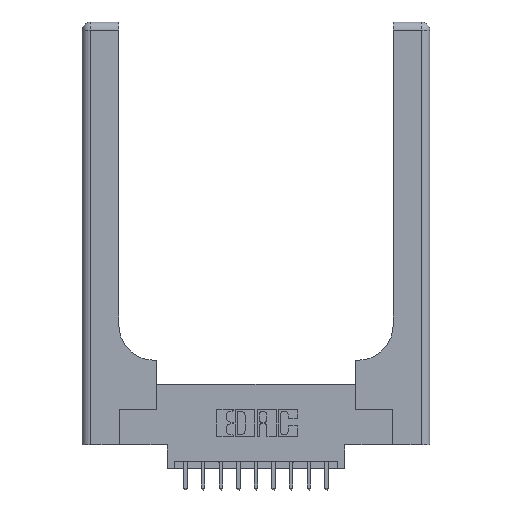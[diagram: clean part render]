
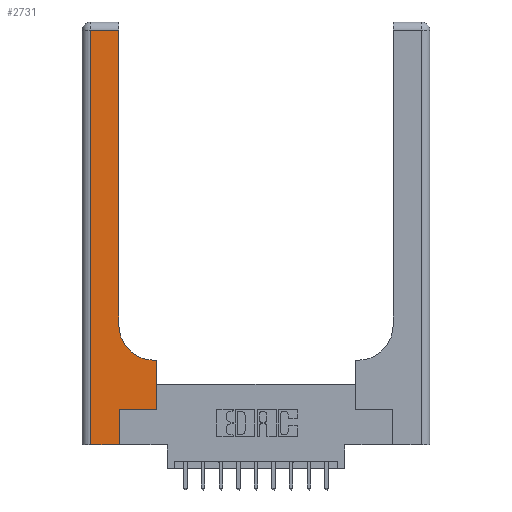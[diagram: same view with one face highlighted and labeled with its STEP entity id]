
A CAD part, top view. The second image highlights one B-rep face of the part: STEP entity #2731.
In plain terms, the highlighted planar face has unit normal (0, 0, 1).
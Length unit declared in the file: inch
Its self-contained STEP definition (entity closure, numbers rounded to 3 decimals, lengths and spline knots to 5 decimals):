
#89 = DIRECTION ( 'NONE',  ( 1., 0., 0. ) ) ;
#247 = CARTESIAN_POINT ( 'NONE',  ( 0.51, 0.85, 0.37 ) ) ;
#337 = VECTOR ( 'NONE', #2389, 39.37008 ) ;
#492 = LINE ( 'NONE', #6686, #12989 ) ;
#712 = EDGE_CURVE ( 'NONE', #7349, #15351, #12527, .T. ) ;
#762 = EDGE_CURVE ( 'NONE', #5859, #15444, #8938, .T. ) ;
#1408 = VECTOR ( 'NONE', #10442, 39.37008 ) ;
#1479 = CARTESIAN_POINT ( 'NONE',  ( 0.265, 0.25, 0.37 ) ) ;
#1550 = LINE ( 'NONE', #6518, #12746 ) ;
#1628 = VECTOR ( 'NONE', #10162, 39.37008 ) ;
#1640 = LINE ( 'NONE', #9027, #1628 ) ;
#1655 = ORIENTED_EDGE ( 'NONE', *, *, #3115, .T. ) ;
#1738 = VERTEX_POINT ( 'NONE', #7771 ) ;
#1803 = LINE ( 'NONE', #6767, #12685 ) ;
#2389 = DIRECTION ( 'NONE',  ( 0., 1., 0. ) ) ;
#2731 = ADVANCED_FACE ( 'NONE', ( #12459 ), #4994, .F. ) ;
#3050 = ORIENTED_EDGE ( 'NONE', *, *, #10567, .T. ) ;
#3115 = EDGE_CURVE ( 'NONE', #15982, #5859, #492, .T. ) ;
#3311 = LINE ( 'NONE', #5437, #1408 ) ;
#3332 = ORIENTED_EDGE ( 'NONE', *, *, #15633, .T. ) ;
#3412 = ORIENTED_EDGE ( 'NONE', *, *, #13233, .T. ) ;
#4410 = VERTEX_POINT ( 'NONE', #16093 ) ;
#4531 = ORIENTED_EDGE ( 'NONE', *, *, #712, .T. ) ;
#4686 = ORIENTED_EDGE ( 'NONE', *, *, #762, .T. ) ;
#4962 = AXIS2_PLACEMENT_3D ( 'NONE', #8559, #8634, #7187 ) ;
#4994 = PLANE ( 'NONE',  #4962 ) ;
#5211 = LINE ( 'NONE', #6184, #6594 ) ;
#5437 = CARTESIAN_POINT ( 'NONE',  ( 0.528, 0.25, 0.37 ) ) ;
#5447 = EDGE_CURVE ( 'NONE', #1738, #7543, #1803, .T. ) ;
#5859 = VERTEX_POINT ( 'NONE', #10223 ) ;
#5895 = CARTESIAN_POINT ( 'NONE',  ( 0.265, 0., 0.37 ) ) ;
#6066 = ORIENTED_EDGE ( 'NONE', *, *, #5447, .T. ) ;
#6184 = CARTESIAN_POINT ( 'NONE',  ( 0., 2.94, 0.37 ) ) ;
#6518 = CARTESIAN_POINT ( 'NONE',  ( 0.26, 3., 0.37 ) ) ;
#6594 = VECTOR ( 'NONE', #10142, 39.37008 ) ;
#6686 = CARTESIAN_POINT ( 'NONE',  ( 0.26, 0.6, 0.37 ) ) ;
#6743 = CARTESIAN_POINT ( 'NONE',  ( 0.265, 0., 0.37 ) ) ;
#6767 = CARTESIAN_POINT ( 'NONE',  ( 0., 0., 0.37 ) ) ;
#7039 = EDGE_LOOP ( 'NONE', ( #3050, #8176, #14363, #6066, #3412, #4531, #3332, #1655, #4686 ) ) ;
#7187 = DIRECTION ( 'NONE',  ( -1., 0., 0. ) ) ;
#7349 = VERTEX_POINT ( 'NONE', #8544 ) ;
#7538 = VERTEX_POINT ( 'NONE', #11926 ) ;
#7543 = VERTEX_POINT ( 'NONE', #6743 ) ;
#7771 = CARTESIAN_POINT ( 'NONE',  ( 0.06, 0., 0.37 ) ) ;
#8176 = ORIENTED_EDGE ( 'NONE', *, *, #13588, .T. ) ;
#8544 = CARTESIAN_POINT ( 'NONE',  ( 0.265, 0.25, 0.37 ) ) ;
#8559 = CARTESIAN_POINT ( 'NONE',  ( 0., 3., 0.37 ) ) ;
#8634 = DIRECTION ( 'NONE',  ( 0., 0., -1. ) ) ;
#8719 = EDGE_CURVE ( 'NONE', #7538, #1738, #1640, .T. ) ;
#8938 = CIRCLE ( 'NONE', #12840, 0.25 ) ;
#9027 = CARTESIAN_POINT ( 'NONE',  ( 0.06, 3., 0.37 ) ) ;
#10078 = DIRECTION ( 'NONE',  ( 0., 0., -1. ) ) ;
#10142 = DIRECTION ( 'NONE',  ( -1., 0., 0. ) ) ;
#10162 = DIRECTION ( 'NONE',  ( 0., -1., 0. ) ) ;
#10223 = CARTESIAN_POINT ( 'NONE',  ( 0.51, 0.6, 0.37 ) ) ;
#10442 = DIRECTION ( 'NONE',  ( 0., 1., 0. ) ) ;
#10567 = EDGE_CURVE ( 'NONE', #15444, #4410, #1550, .T. ) ;
#11039 = CARTESIAN_POINT ( 'NONE',  ( 0.26, 0.85, 0.37 ) ) ;
#11446 = DIRECTION ( 'NONE',  ( 0., 1., 0. ) ) ;
#11621 = DIRECTION ( 'NONE',  ( -1., 0., 0. ) ) ;
#11704 = DIRECTION ( 'NONE',  ( 1., 0., 0. ) ) ;
#11779 = VECTOR ( 'NONE', #89, 39.37008 ) ;
#11926 = CARTESIAN_POINT ( 'NONE',  ( 0.06, 2.94, 0.37 ) ) ;
#12459 = FACE_OUTER_BOUND ( 'NONE', #7039, .T. ) ;
#12527 = LINE ( 'NONE', #1479, #11779 ) ;
#12685 = VECTOR ( 'NONE', #11704, 39.37008 ) ;
#12746 = VECTOR ( 'NONE', #11446, 39.37008 ) ;
#12840 = AXIS2_PLACEMENT_3D ( 'NONE', #247, #10078, #15058 ) ;
#12989 = VECTOR ( 'NONE', #11621, 39.37008 ) ;
#13233 = EDGE_CURVE ( 'NONE', #7543, #7349, #13520, .T. ) ;
#13270 = CARTESIAN_POINT ( 'NONE',  ( 0.528, 0.6, 0.37 ) ) ;
#13520 = LINE ( 'NONE', #5895, #337 ) ;
#13588 = EDGE_CURVE ( 'NONE', #4410, #7538, #5211, .T. ) ;
#14363 = ORIENTED_EDGE ( 'NONE', *, *, #8719, .T. ) ;
#14803 = CARTESIAN_POINT ( 'NONE',  ( 0.528, 0.25, 0.37 ) ) ;
#15058 = DIRECTION ( 'NONE',  ( 1., 0., 0. ) ) ;
#15351 = VERTEX_POINT ( 'NONE', #14803 ) ;
#15444 = VERTEX_POINT ( 'NONE', #11039 ) ;
#15633 = EDGE_CURVE ( 'NONE', #15351, #15982, #3311, .T. ) ;
#15982 = VERTEX_POINT ( 'NONE', #13270 ) ;
#16093 = CARTESIAN_POINT ( 'NONE',  ( 0.26, 2.94, 0.37 ) ) ;
